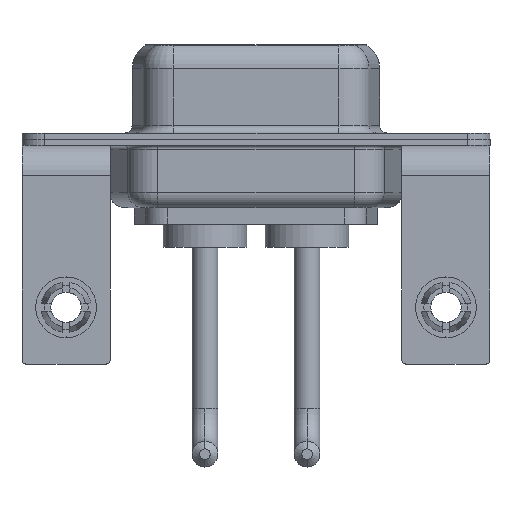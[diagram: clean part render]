
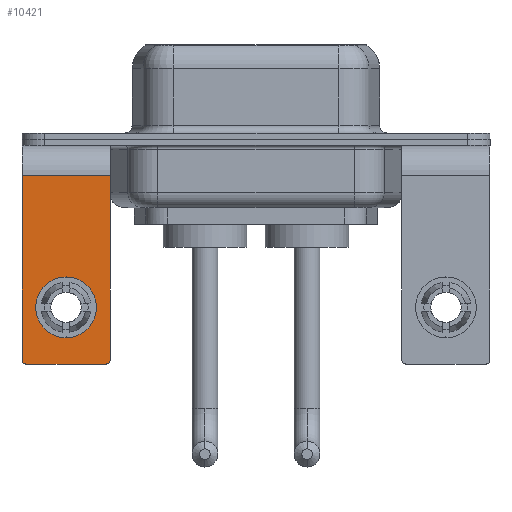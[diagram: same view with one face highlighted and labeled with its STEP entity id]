
A CAD part, front view. The second image highlights one B-rep face of the part: STEP entity #10421.
In plain terms, the highlighted planar face has unit normal (0, -1, 0).
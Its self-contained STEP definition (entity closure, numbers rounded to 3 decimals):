
#628 = DIRECTION ( 'NONE',  ( 0., 1., 0. ) ) ;
#691 = DIRECTION ( 'NONE',  ( 0., 0., 1. ) ) ;
#900 = PLANE ( 'NONE',  #1743 ) ;
#941 = CIRCLE ( 'NONE', #3532, 2. ) ;
#1088 = VERTEX_POINT ( 'NONE', #13058 ) ;
#1238 = EDGE_CURVE ( 'NONE', #6033, #1088, #10249, .T. ) ;
#1358 = CARTESIAN_POINT ( 'NONE',  ( 2.65, -6.25, -14.8 ) ) ;
#1359 = AXIS2_PLACEMENT_3D ( 'NONE', #4056, #2879, #8546 ) ;
#1743 = AXIS2_PLACEMENT_3D ( 'NONE', #14225, #628, #4150 ) ;
#2101 = ORIENTED_EDGE ( 'NONE', *, *, #11674, .T. ) ;
#2234 = DIRECTION ( 'NONE',  ( -1., 0., 0. ) ) ;
#2313 = CARTESIAN_POINT ( 'NONE',  ( 2.9, -6.25, -2.4 ) ) ;
#2485 = LINE ( 'NONE', #5799, #11967 ) ;
#2879 = DIRECTION ( 'NONE',  ( 0., -1., 0. ) ) ;
#2882 = CIRCLE ( 'NONE', #12736, 2. ) ;
#3175 = DIRECTION ( 'NONE',  ( 0., 0., 1. ) ) ;
#3532 = AXIS2_PLACEMENT_3D ( 'NONE', #10772, #9955, #691 ) ;
#4056 = CARTESIAN_POINT ( 'NONE',  ( -2.65, -6.25, -14.55 ) ) ;
#4150 = DIRECTION ( 'NONE',  ( 0., 0., 1. ) ) ;
#4175 = EDGE_CURVE ( 'NONE', #7553, #6369, #2485, .T. ) ;
#4774 = CARTESIAN_POINT ( 'NONE',  ( -2.9, -6.25, -2.4 ) ) ;
#4833 = VECTOR ( 'NONE', #4999, 1000. ) ;
#4848 = DIRECTION ( 'NONE',  ( 0., 0., 1. ) ) ;
#4999 = DIRECTION ( 'NONE',  ( -1., 0., 0. ) ) ;
#5263 = ORIENTED_EDGE ( 'NONE', *, *, #8872, .T. ) ;
#5335 = ORIENTED_EDGE ( 'NONE', *, *, #1238, .F. ) ;
#5574 = EDGE_LOOP ( 'NONE', ( #11981, #2101, #5335, #11766, #13069, #9826 ) ) ;
#5784 = CIRCLE ( 'NONE', #6265, 0.25 ) ;
#5799 = CARTESIAN_POINT ( 'NONE',  ( -2.9, -6.25, -2.4 ) ) ;
#5959 = CARTESIAN_POINT ( 'NONE',  ( 2.9, -6.25, -2.4 ) ) ;
#6033 = VERTEX_POINT ( 'NONE', #1358 ) ;
#6265 = AXIS2_PLACEMENT_3D ( 'NONE', #7593, #9654, #3175 ) ;
#6345 = VERTEX_POINT ( 'NONE', #12035 ) ;
#6369 = VERTEX_POINT ( 'NONE', #13133 ) ;
#6789 = EDGE_CURVE ( 'NONE', #10336, #9271, #941, .T. ) ;
#6800 = DIRECTION ( 'NONE',  ( 0., 0., -1. ) ) ;
#7269 = CARTESIAN_POINT ( 'NONE',  ( 0., -6.25, -13.07 ) ) ;
#7374 = VERTEX_POINT ( 'NONE', #13520 ) ;
#7553 = VERTEX_POINT ( 'NONE', #4774 ) ;
#7593 = CARTESIAN_POINT ( 'NONE',  ( 2.65, -6.25, -14.55 ) ) ;
#7665 = VECTOR ( 'NONE', #6800, 1000. ) ;
#8430 = CIRCLE ( 'NONE', #1359, 0.25 ) ;
#8546 = DIRECTION ( 'NONE',  ( 0., 0., 1. ) ) ;
#8665 = ORIENTED_EDGE ( 'NONE', *, *, #6789, .T. ) ;
#8872 = EDGE_CURVE ( 'NONE', #9271, #10336, #2882, .T. ) ;
#9037 = DIRECTION ( 'NONE',  ( 0., 0., -1. ) ) ;
#9271 = VERTEX_POINT ( 'NONE', #7269 ) ;
#9422 = LINE ( 'NONE', #5959, #4833 ) ;
#9654 = DIRECTION ( 'NONE',  ( 0., -1., 0. ) ) ;
#9826 = ORIENTED_EDGE ( 'NONE', *, *, #11524, .T. ) ;
#9955 = DIRECTION ( 'NONE',  ( 0., 1., 0. ) ) ;
#10240 = VECTOR ( 'NONE', #2234, 1000. ) ;
#10249 = LINE ( 'NONE', #13557, #10240 ) ;
#10336 = VERTEX_POINT ( 'NONE', #14302 ) ;
#10421 = ADVANCED_FACE ( 'NONE', ( #10986, #10704 ), #900, .F. ) ;
#10446 = DIRECTION ( 'NONE',  ( 0., 1., 0. ) ) ;
#10704 = FACE_OUTER_BOUND ( 'NONE', #5574, .T. ) ;
#10772 = CARTESIAN_POINT ( 'NONE',  ( 0., -6.25, -11.07 ) ) ;
#10986 = FACE_BOUND ( 'NONE', #14274, .T. ) ;
#11524 = EDGE_CURVE ( 'NONE', #7374, #7553, #9422, .T. ) ;
#11674 = EDGE_CURVE ( 'NONE', #6369, #1088, #8430, .T. ) ;
#11766 = ORIENTED_EDGE ( 'NONE', *, *, #14454, .T. ) ;
#11967 = VECTOR ( 'NONE', #9037, 1000. ) ;
#11981 = ORIENTED_EDGE ( 'NONE', *, *, #4175, .T. ) ;
#12035 = CARTESIAN_POINT ( 'NONE',  ( 2.9, -6.25, -14.55 ) ) ;
#12396 = LINE ( 'NONE', #2313, #7665 ) ;
#12577 = CARTESIAN_POINT ( 'NONE',  ( 0., -6.25, -11.07 ) ) ;
#12736 = AXIS2_PLACEMENT_3D ( 'NONE', #12577, #10446, #4848 ) ;
#13058 = CARTESIAN_POINT ( 'NONE',  ( -2.65, -6.25, -14.8 ) ) ;
#13069 = ORIENTED_EDGE ( 'NONE', *, *, #13804, .F. ) ;
#13133 = CARTESIAN_POINT ( 'NONE',  ( -2.9, -6.25, -14.55 ) ) ;
#13520 = CARTESIAN_POINT ( 'NONE',  ( 2.9, -6.25, -2.4 ) ) ;
#13557 = CARTESIAN_POINT ( 'NONE',  ( 2.9, -6.25, -14.8 ) ) ;
#13804 = EDGE_CURVE ( 'NONE', #7374, #6345, #12396, .T. ) ;
#14225 = CARTESIAN_POINT ( 'NONE',  ( 2.9, -6.25, -2.4 ) ) ;
#14274 = EDGE_LOOP ( 'NONE', ( #5263, #8665 ) ) ;
#14302 = CARTESIAN_POINT ( 'NONE',  ( 0., -6.25, -9.07 ) ) ;
#14454 = EDGE_CURVE ( 'NONE', #6033, #6345, #5784, .T. ) ;
